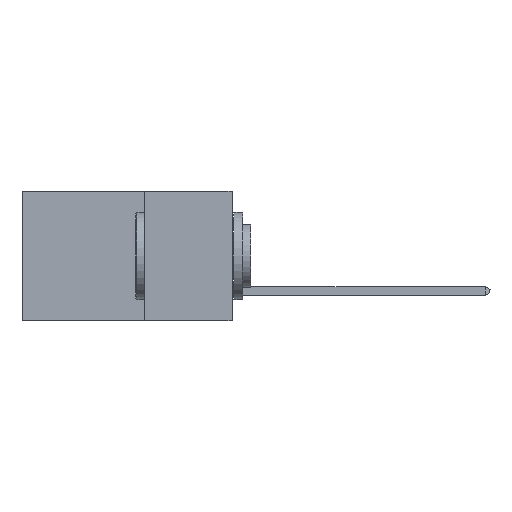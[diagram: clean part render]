
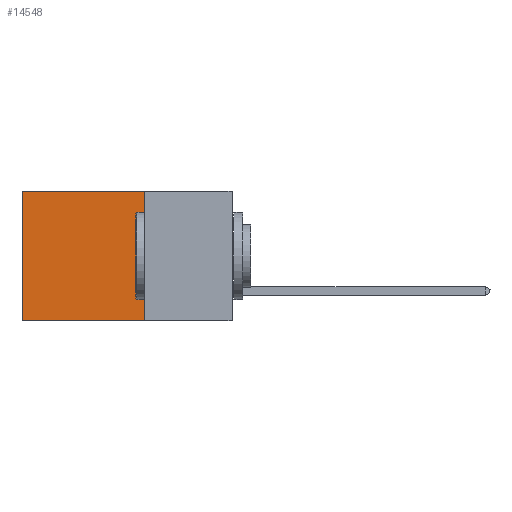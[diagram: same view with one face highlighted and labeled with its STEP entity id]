
A CAD part, left-side view. The second image highlights one B-rep face of the part: STEP entity #14548.
In plain terms, the highlighted planar face has unit normal (-1, 0, 0).
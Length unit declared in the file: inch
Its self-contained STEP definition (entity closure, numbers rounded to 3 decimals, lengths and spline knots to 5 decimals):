
#1468 = VERTEX_POINT ( 'NONE', #16019 ) ;
#2748 = VERTEX_POINT ( 'NONE', #26591 ) ;
#3077 = VECTOR ( 'NONE', #43292, 39.37008 ) ;
#4317 = LINE ( 'NONE', #35071, #13984 ) ;
#7189 = CARTESIAN_POINT ( 'NONE',  ( 0.2875, 0.25, 0. ) ) ;
#7825 = ORIENTED_EDGE ( 'NONE', *, *, #21236, .T. ) ;
#8283 = DIRECTION ( 'NONE',  ( 1., 0., 0. ) ) ;
#11775 = CARTESIAN_POINT ( 'NONE',  ( 0.2875, 0.25, 0. ) ) ;
#13984 = VECTOR ( 'NONE', #28219, 39.37008 ) ;
#14548 = ADVANCED_FACE ( 'NONE', ( #16004 ), #25904, .F. ) ;
#15542 = EDGE_CURVE ( 'NONE', #1468, #41440, #34187, .T. ) ;
#16004 = FACE_OUTER_BOUND ( 'NONE', #31389, .T. ) ;
#16019 = CARTESIAN_POINT ( 'NONE',  ( 0.2875, 0.25, 0. ) ) ;
#16537 = ORIENTED_EDGE ( 'NONE', *, *, #15542, .F. ) ;
#20687 = DIRECTION ( 'NONE',  ( 0., 1., 0. ) ) ;
#21236 = EDGE_CURVE ( 'NONE', #1468, #2748, #44163, .T. ) ;
#21878 = EDGE_CURVE ( 'NONE', #2748, #35335, #4317, .T. ) ;
#22539 = DIRECTION ( 'NONE',  ( 0., 0., -1. ) ) ;
#24070 = AXIS2_PLACEMENT_3D ( 'NONE', #11775, #8283, #22539 ) ;
#24342 = LINE ( 'NONE', #32319, #43847 ) ;
#24412 = DIRECTION ( 'NONE',  ( 0., 1., 0. ) ) ;
#25092 = EDGE_CURVE ( 'NONE', #41440, #35335, #24342, .T. ) ;
#25499 = CARTESIAN_POINT ( 'NONE',  ( 0.2875, 0.25, -0.37 ) ) ;
#25904 = PLANE ( 'NONE',  #24070 ) ;
#26591 = CARTESIAN_POINT ( 'NONE',  ( 0.2875, 0.6, 0. ) ) ;
#28219 = DIRECTION ( 'NONE',  ( 0., 0., -1. ) ) ;
#29003 = VECTOR ( 'NONE', #20687, 39.37008 ) ;
#31389 = EDGE_LOOP ( 'NONE', ( #43686, #36395, #16537, #7825 ) ) ;
#32319 = CARTESIAN_POINT ( 'NONE',  ( 0.2875, 0.25, -0.37 ) ) ;
#34187 = LINE ( 'NONE', #36200, #3077 ) ;
#34252 = CARTESIAN_POINT ( 'NONE',  ( 0.2875, 0.6, -0.37 ) ) ;
#35071 = CARTESIAN_POINT ( 'NONE',  ( 0.2875, 0.6, 0. ) ) ;
#35335 = VERTEX_POINT ( 'NONE', #34252 ) ;
#36200 = CARTESIAN_POINT ( 'NONE',  ( 0.2875, 0.25, 0. ) ) ;
#36395 = ORIENTED_EDGE ( 'NONE', *, *, #25092, .F. ) ;
#41440 = VERTEX_POINT ( 'NONE', #25499 ) ;
#43292 = DIRECTION ( 'NONE',  ( 0., 0., -1. ) ) ;
#43686 = ORIENTED_EDGE ( 'NONE', *, *, #21878, .T. ) ;
#43847 = VECTOR ( 'NONE', #24412, 39.37008 ) ;
#44163 = LINE ( 'NONE', #7189, #29003 ) ;
